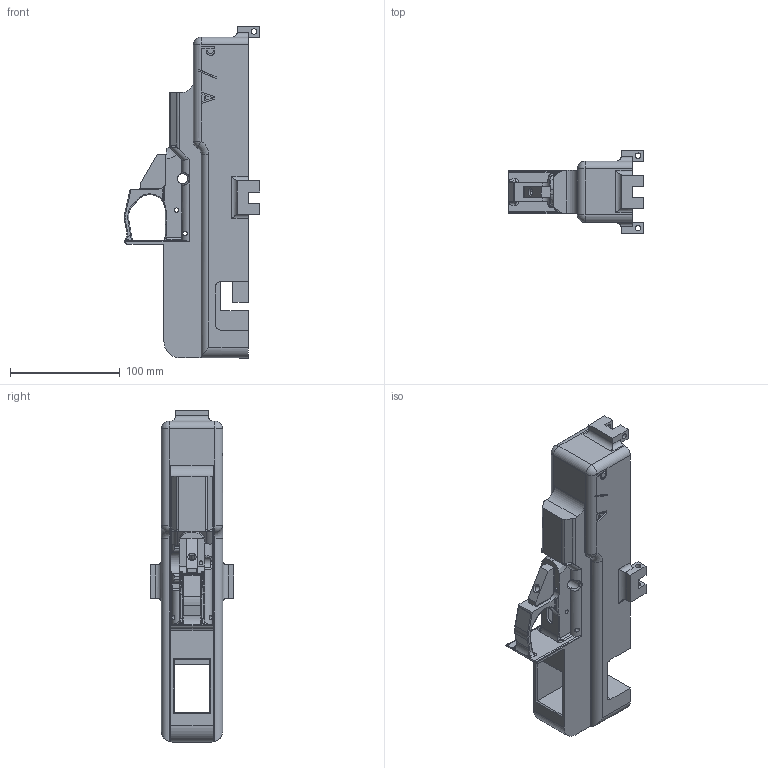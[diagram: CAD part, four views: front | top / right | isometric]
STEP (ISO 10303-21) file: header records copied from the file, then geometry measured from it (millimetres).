
FILE_DESCRIPTION (( 'STEP AP214' ), '1' );
FILE_NAME ('Frame_pre_real.STEP', '2013-09-28T02:33:47', ( '' ), ( '' ), 'SwSTEP 2.0', 'SolidWorks 2013', '' );
FILE_SCHEMA (( 'AUTOMOTIVE_DESIGN' ));
Length unit declared in the file: millimetre
Products named in the file (1): Frame_pre_real
Bounding box: 123.33 x 76.25 x 303 mm (x, y, z)
Volume: 523190.5 mm3; surface area: 123786 mm2
Topology: 1 solids, 1 shells, 404 faces, 1102 edges, 695 vertices
Faces by surface type: plane 172, cylinder 153, bspline 58, torus 13, cone 4, sphere 4
Entity records: 15963 total; most frequent: CARTESIAN_POINT 6119, ORIENTED_EDGE 2196, DIRECTION 1878, EDGE_CURVE 1098, VERTEX_POINT 695, AXIS2_PLACEMENT_3D 631, LINE 616, VECTOR 616
